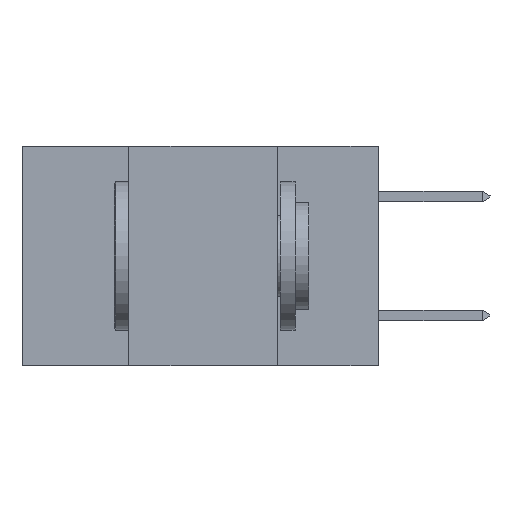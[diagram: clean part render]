
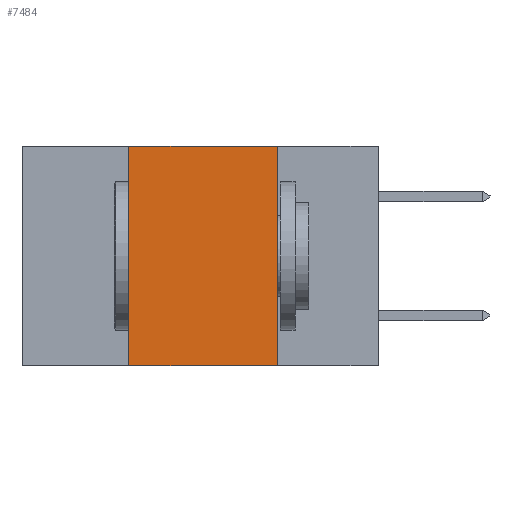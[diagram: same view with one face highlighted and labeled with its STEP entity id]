
A CAD part, left-side view. The second image highlights one B-rep face of the part: STEP entity #7484.
In plain terms, the highlighted planar face has unit normal (-1, 0, 0).
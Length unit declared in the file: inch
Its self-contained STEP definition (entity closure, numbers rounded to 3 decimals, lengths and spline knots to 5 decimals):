
#349 = CARTESIAN_POINT ( 'NONE',  ( 0., 0.42, -0.37 ) ) ;
#578 = ORIENTED_EDGE ( 'NONE', *, *, #9512, .F. ) ;
#1409 = PLANE ( 'NONE',  #2224 ) ;
#2093 = EDGE_LOOP ( 'NONE', ( #3156, #8006, #578, #19909 ) ) ;
#2224 = AXIS2_PLACEMENT_3D ( 'NONE', #2859, #7346, #10890 ) ;
#2243 = VERTEX_POINT ( 'NONE', #14437 ) ;
#2859 = CARTESIAN_POINT ( 'NONE',  ( 0., 0.6, 0. ) ) ;
#3102 = VECTOR ( 'NONE', #23883, 39.37008 ) ;
#3156 = ORIENTED_EDGE ( 'NONE', *, *, #23760, .F. ) ;
#4157 = LINE ( 'NONE', #349, #22730 ) ;
#4637 = DIRECTION ( 'NONE',  ( 0., -1., 0. ) ) ;
#5783 = DIRECTION ( 'NONE',  ( 0., 0., -1. ) ) ;
#5944 = CARTESIAN_POINT ( 'NONE',  ( 0., 0.6, -0.37 ) ) ;
#6059 = VECTOR ( 'NONE', #5783, 39.37008 ) ;
#6165 = CARTESIAN_POINT ( 'NONE',  ( 0., 0.42, 0. ) ) ;
#7346 = DIRECTION ( 'NONE',  ( 1., 0., 0. ) ) ;
#7484 = ADVANCED_FACE ( 'NONE', ( #20816 ), #1409, .F. ) ;
#8006 = ORIENTED_EDGE ( 'NONE', *, *, #12687, .F. ) ;
#8372 = DIRECTION ( 'NONE',  ( 0., 0., 1. ) ) ;
#9350 = LINE ( 'NONE', #17307, #6059 ) ;
#9512 = EDGE_CURVE ( 'NONE', #2243, #13194, #4157, .T. ) ;
#10346 = EDGE_CURVE ( 'NONE', #2243, #21305, #20444, .T. ) ;
#10890 = DIRECTION ( 'NONE',  ( 0., 0., -1. ) ) ;
#11110 = CARTESIAN_POINT ( 'NONE',  ( 0., 0.17, -0.37 ) ) ;
#12512 = CARTESIAN_POINT ( 'NONE',  ( 0., 0.6, 0. ) ) ;
#12687 = EDGE_CURVE ( 'NONE', #13194, #13229, #14471, .T. ) ;
#13194 = VERTEX_POINT ( 'NONE', #6165 ) ;
#13229 = VERTEX_POINT ( 'NONE', #18191 ) ;
#14437 = CARTESIAN_POINT ( 'NONE',  ( 0., 0.42, -0.37 ) ) ;
#14471 = LINE ( 'NONE', #12512, #19347 ) ;
#17307 = CARTESIAN_POINT ( 'NONE',  ( 0., 0.17, -0.37 ) ) ;
#18191 = CARTESIAN_POINT ( 'NONE',  ( 0., 0.17, 0. ) ) ;
#19347 = VECTOR ( 'NONE', #4637, 39.37008 ) ;
#19909 = ORIENTED_EDGE ( 'NONE', *, *, #10346, .T. ) ;
#20444 = LINE ( 'NONE', #5944, #3102 ) ;
#20816 = FACE_OUTER_BOUND ( 'NONE', #2093, .T. ) ;
#21305 = VERTEX_POINT ( 'NONE', #11110 ) ;
#22730 = VECTOR ( 'NONE', #8372, 39.37008 ) ;
#23760 = EDGE_CURVE ( 'NONE', #13229, #21305, #9350, .T. ) ;
#23883 = DIRECTION ( 'NONE',  ( 0., -1., 0. ) ) ;
